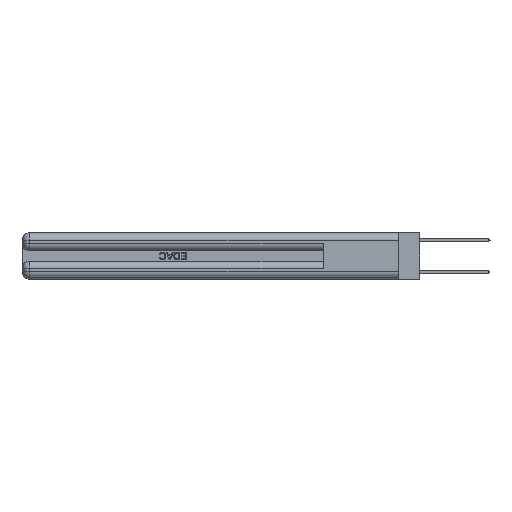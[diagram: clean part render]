
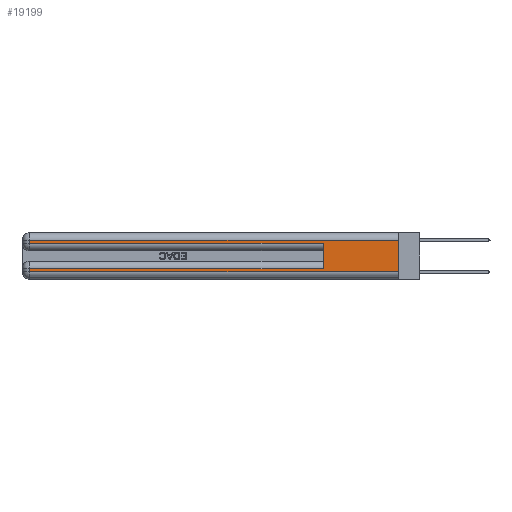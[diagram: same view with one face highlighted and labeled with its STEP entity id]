
A CAD part, left-side view. The second image highlights one B-rep face of the part: STEP entity #19199.
In plain terms, the highlighted planar face has unit normal (-1, 0, 0).
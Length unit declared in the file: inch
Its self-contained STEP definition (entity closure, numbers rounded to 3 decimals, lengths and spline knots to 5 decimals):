
#111 = EDGE_CURVE ( 'NONE', #31182, #27999, #19333, .T. ) ;
#573 = PLANE ( 'NONE',  #24861 ) ;
#1565 = ORIENTED_EDGE ( 'NONE', *, *, #15430, .T. ) ;
#2062 = VECTOR ( 'NONE', #30803, 39.37008 ) ;
#2292 = FACE_OUTER_BOUND ( 'NONE', #18641, .T. ) ;
#2885 = LINE ( 'NONE', #15177, #2062 ) ;
#3121 = CARTESIAN_POINT ( 'NONE',  ( 0., 0., 0.37 ) ) ;
#3195 = VECTOR ( 'NONE', #27533, 39.37008 ) ;
#3235 = DIRECTION ( 'NONE',  ( 0., 0., -1. ) ) ;
#3535 = DIRECTION ( 'NONE',  ( 0., 1., 0. ) ) ;
#3898 = CARTESIAN_POINT ( 'NONE',  ( 0., 2.94, 0.37 ) ) ;
#4500 = ORIENTED_EDGE ( 'NONE', *, *, #12359, .T. ) ;
#4925 = CARTESIAN_POINT ( 'NONE',  ( 0., 0., 0.085 ) ) ;
#4972 = LINE ( 'NONE', #23160, #18015 ) ;
#5453 = VECTOR ( 'NONE', #25802, 39.37008 ) ;
#5479 = LINE ( 'NONE', #16513, #25470 ) ;
#6173 = CARTESIAN_POINT ( 'NONE',  ( 0., 0., 0.31 ) ) ;
#6516 = DIRECTION ( 'NONE',  ( 0., 0., -1. ) ) ;
#6885 = VERTEX_POINT ( 'NONE', #16576 ) ;
#8057 = CARTESIAN_POINT ( 'NONE',  ( 0., 0.6, 0.085 ) ) ;
#8900 = EDGE_CURVE ( 'NONE', #27999, #6885, #17890, .T. ) ;
#10806 = CARTESIAN_POINT ( 'NONE',  ( 0., 2.94, 0.285 ) ) ;
#12359 = EDGE_CURVE ( 'NONE', #6885, #21508, #5479, .T. ) ;
#13049 = ORIENTED_EDGE ( 'NONE', *, *, #8900, .T. ) ;
#13927 = VERTEX_POINT ( 'NONE', #18024 ) ;
#15177 = CARTESIAN_POINT ( 'NONE',  ( 0., 0., 0.37 ) ) ;
#15430 = EDGE_CURVE ( 'NONE', #23162, #18320, #4972, .T. ) ;
#16513 = CARTESIAN_POINT ( 'NONE',  ( 0., 0., 0.06 ) ) ;
#16542 = EDGE_CURVE ( 'NONE', #22728, #21508, #2885, .T. ) ;
#16576 = CARTESIAN_POINT ( 'NONE',  ( 0., 2.94, 0.06 ) ) ;
#16639 = CARTESIAN_POINT ( 'NONE',  ( 0., 0., 0.31 ) ) ;
#17890 = LINE ( 'NONE', #30127, #3195 ) ;
#17891 = CARTESIAN_POINT ( 'NONE',  ( 0., 0.6, 0.285 ) ) ;
#18015 = VECTOR ( 'NONE', #18016, 39.37008 ) ;
#18016 = DIRECTION ( 'NONE',  ( 0., -1., 0. ) ) ;
#18024 = CARTESIAN_POINT ( 'NONE',  ( 0., 2.94, 0.31 ) ) ;
#18320 = VERTEX_POINT ( 'NONE', #17891 ) ;
#18641 = EDGE_LOOP ( 'NONE', ( #21560, #31307, #18730, #1565, #33490, #25741, #13049, #4500 ) ) ;
#18730 = ORIENTED_EDGE ( 'NONE', *, *, #19790, .T. ) ;
#18877 = DIRECTION ( 'NONE',  ( 1., 0., 0. ) ) ;
#19199 = ADVANCED_FACE ( 'NONE', ( #2292 ), #573, .F. ) ;
#19333 = LINE ( 'NONE', #4925, #5453 ) ;
#19591 = CARTESIAN_POINT ( 'NONE',  ( 0., 0., 0.06 ) ) ;
#19790 = EDGE_CURVE ( 'NONE', #13927, #23162, #25957, .T. ) ;
#21508 = VERTEX_POINT ( 'NONE', #19591 ) ;
#21560 = ORIENTED_EDGE ( 'NONE', *, *, #16542, .F. ) ;
#21729 = CARTESIAN_POINT ( 'NONE',  ( 0., 2.94, 0.085 ) ) ;
#21770 = DIRECTION ( 'NONE',  ( 0., -1., 0. ) ) ;
#21880 = LINE ( 'NONE', #22095, #27993 ) ;
#22095 = CARTESIAN_POINT ( 'NONE',  ( 0., 0.6, 0.145 ) ) ;
#22141 = VECTOR ( 'NONE', #3535, 39.37008 ) ;
#22728 = VERTEX_POINT ( 'NONE', #6173 ) ;
#22954 = LINE ( 'NONE', #16639, #22141 ) ;
#23160 = CARTESIAN_POINT ( 'NONE',  ( 0., 0., 0.285 ) ) ;
#23162 = VERTEX_POINT ( 'NONE', #10806 ) ;
#24861 = AXIS2_PLACEMENT_3D ( 'NONE', #3121, #18877, #3235 ) ;
#25470 = VECTOR ( 'NONE', #21770, 39.37008 ) ;
#25741 = ORIENTED_EDGE ( 'NONE', *, *, #111, .T. ) ;
#25802 = DIRECTION ( 'NONE',  ( 0., 1., 0. ) ) ;
#25957 = LINE ( 'NONE', #3898, #32064 ) ;
#26604 = EDGE_CURVE ( 'NONE', #22728, #13927, #22954, .T. ) ;
#27533 = DIRECTION ( 'NONE',  ( 0., 0., -1. ) ) ;
#27993 = VECTOR ( 'NONE', #29951, 39.37008 ) ;
#27999 = VERTEX_POINT ( 'NONE', #21729 ) ;
#29433 = EDGE_CURVE ( 'NONE', #31182, #18320, #21880, .T. ) ;
#29951 = DIRECTION ( 'NONE',  ( 0., 0., 1. ) ) ;
#30127 = CARTESIAN_POINT ( 'NONE',  ( 0., 2.94, 0.37 ) ) ;
#30803 = DIRECTION ( 'NONE',  ( 0., 0., -1. ) ) ;
#31182 = VERTEX_POINT ( 'NONE', #8057 ) ;
#31307 = ORIENTED_EDGE ( 'NONE', *, *, #26604, .T. ) ;
#32064 = VECTOR ( 'NONE', #6516, 39.37008 ) ;
#33490 = ORIENTED_EDGE ( 'NONE', *, *, #29433, .F. ) ;
